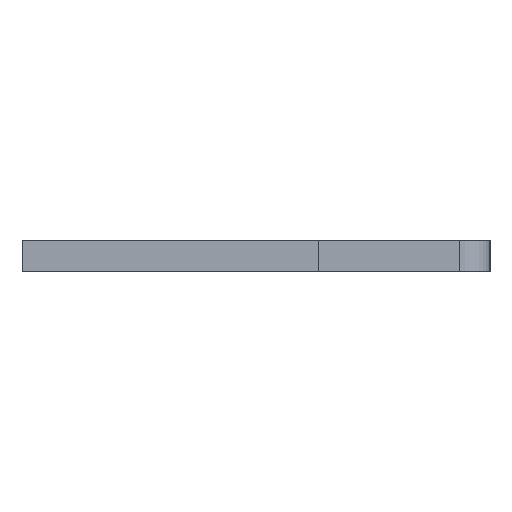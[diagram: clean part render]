
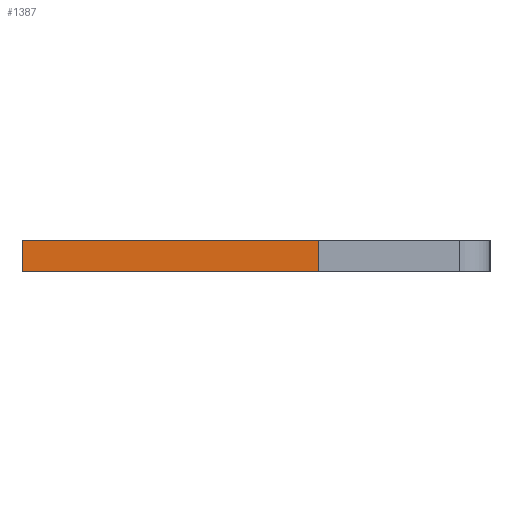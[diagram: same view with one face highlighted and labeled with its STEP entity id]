
A CAD part, left-side view. The second image highlights one B-rep face of the part: STEP entity #1387.
In plain terms, the highlighted face is planar.
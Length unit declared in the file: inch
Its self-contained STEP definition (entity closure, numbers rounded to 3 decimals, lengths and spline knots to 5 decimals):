
#2 = FACE_OUTER_BOUND ( 'NONE', #76, .T. ) ;
#18 = ORIENTED_EDGE ( 'NONE', *, *, #334, .F. ) ;
#76 = EDGE_LOOP ( 'NONE', ( #1413, #249, #18, #95 ) ) ;
#80 = PLANE ( 'NONE',  #425 ) ;
#95 = ORIENTED_EDGE ( 'NONE', *, *, #534, .T. ) ;
#147 = EDGE_CURVE ( 'NONE', #573, #1165, #1732, .T. ) ;
#185 = VERTEX_POINT ( 'NONE', #1173 ) ;
#216 = CARTESIAN_POINT ( 'NONE',  ( -0.01, 0.15, -0.04 ) ) ;
#249 = ORIENTED_EDGE ( 'NONE', *, *, #1375, .F. ) ;
#334 = EDGE_CURVE ( 'NONE', #185, #590, #1593, .T. ) ;
#425 = AXIS2_PLACEMENT_3D ( 'NONE', #1735, #796, #803 ) ;
#534 = EDGE_CURVE ( 'NONE', #185, #573, #1399, .T. ) ;
#542 = DIRECTION ( 'NONE',  ( 0., 1., 0. ) ) ;
#560 = VECTOR ( 'NONE', #878, 39.37008 ) ;
#573 = VERTEX_POINT ( 'NONE', #1066 ) ;
#590 = VERTEX_POINT ( 'NONE', #1512 ) ;
#688 = CARTESIAN_POINT ( 'NONE',  ( -0.01, 0.15, -0.04 ) ) ;
#716 = LINE ( 'NONE', #1753, #1457 ) ;
#796 = DIRECTION ( 'NONE',  ( 0., 0., 1. ) ) ;
#803 = DIRECTION ( 'NONE',  ( 1., 0., 0. ) ) ;
#878 = DIRECTION ( 'NONE',  ( -1., 0., 0. ) ) ;
#888 = DIRECTION ( 'NONE',  ( 0., 1., 0. ) ) ;
#899 = VECTOR ( 'NONE', #542, 39.37008 ) ;
#900 = CARTESIAN_POINT ( 'NONE',  ( 0.01, -0.04, -0.04 ) ) ;
#1045 = CARTESIAN_POINT ( 'NONE',  ( 0.01, 0.15, -0.04 ) ) ;
#1066 = CARTESIAN_POINT ( 'NONE',  ( -0.01, -0.04, -0.04 ) ) ;
#1165 = VERTEX_POINT ( 'NONE', #216 ) ;
#1173 = CARTESIAN_POINT ( 'NONE',  ( 0.01, -0.04, -0.04 ) ) ;
#1375 = EDGE_CURVE ( 'NONE', #590, #1165, #716, .T. ) ;
#1387 = ADVANCED_FACE ( 'NONE', ( #2 ), #80, .F. ) ;
#1399 = LINE ( 'NONE', #900, #560 ) ;
#1413 = ORIENTED_EDGE ( 'NONE', *, *, #147, .T. ) ;
#1457 = VECTOR ( 'NONE', #1751, 39.37008 ) ;
#1512 = CARTESIAN_POINT ( 'NONE',  ( 0.01, 0.15, -0.04 ) ) ;
#1545 = VECTOR ( 'NONE', #888, 39.37008 ) ;
#1593 = LINE ( 'NONE', #1045, #1545 ) ;
#1732 = LINE ( 'NONE', #688, #899 ) ;
#1735 = CARTESIAN_POINT ( 'NONE',  ( 0.01, 0.15, -0.04 ) ) ;
#1751 = DIRECTION ( 'NONE',  ( -1., 0., 0. ) ) ;
#1753 = CARTESIAN_POINT ( 'NONE',  ( 0.01, 0.15, -0.04 ) ) ;
